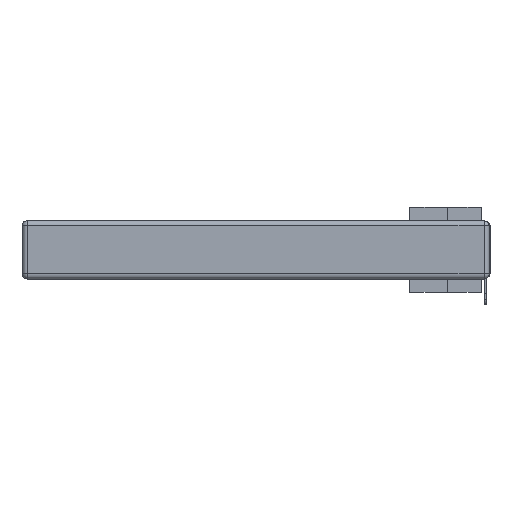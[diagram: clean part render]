
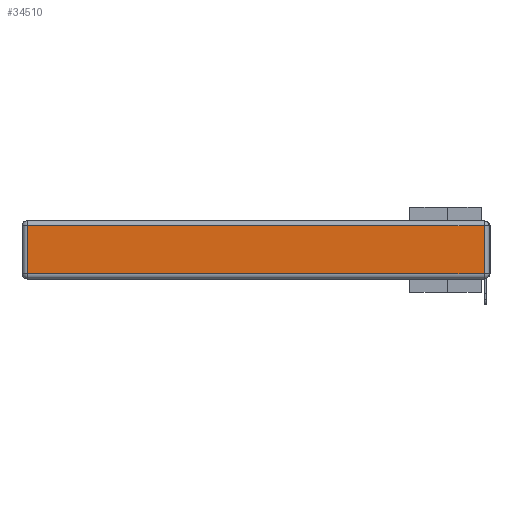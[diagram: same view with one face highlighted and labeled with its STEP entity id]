
A CAD part, left-side view. The second image highlights one B-rep face of the part: STEP entity #34510.
In plain terms, the highlighted planar face has unit normal (-1, 0, 0).
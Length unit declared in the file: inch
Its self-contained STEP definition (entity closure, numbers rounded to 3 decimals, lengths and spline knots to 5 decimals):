
#816 = DIRECTION ( 'NONE',  ( 0., 0., -1. ) ) ;
#1647 = VECTOR ( 'NONE', #14323, 39.37008 ) ;
#2009 = DIRECTION ( 'NONE',  ( 0., -1., 0. ) ) ;
#5439 = EDGE_LOOP ( 'NONE', ( #15310, #11260, #29568, #31312 ) ) ;
#5722 = EDGE_CURVE ( 'NONE', #29702, #23554, #7947, .T. ) ;
#7043 = EDGE_CURVE ( 'NONE', #12979, #22722, #29126, .T. ) ;
#7947 = LINE ( 'NONE', #18188, #13796 ) ;
#8484 = CARTESIAN_POINT ( 'NONE',  ( 0., 0.03, -0.03 ) ) ;
#8891 = CARTESIAN_POINT ( 'NONE',  ( 0., 0., -0.343 ) ) ;
#11260 = ORIENTED_EDGE ( 'NONE', *, *, #16206, .T. ) ;
#11688 = PLANE ( 'NONE',  #19322 ) ;
#12421 = LINE ( 'NONE', #22014, #30352 ) ;
#12979 = VERTEX_POINT ( 'NONE', #8484 ) ;
#13796 = VECTOR ( 'NONE', #2009, 39.37008 ) ;
#14323 = DIRECTION ( 'NONE',  ( 0., 0., 1. ) ) ;
#15310 = ORIENTED_EDGE ( 'NONE', *, *, #5722, .T. ) ;
#16206 = EDGE_CURVE ( 'NONE', #23554, #12979, #17492, .T. ) ;
#17492 = LINE ( 'NONE', #20139, #1647 ) ;
#18188 = CARTESIAN_POINT ( 'NONE',  ( 0., 0., -0.313 ) ) ;
#18224 = DIRECTION ( 'NONE',  ( 0., 1., 0. ) ) ;
#19322 = AXIS2_PLACEMENT_3D ( 'NONE', #8891, #24958, #27906 ) ;
#19706 = CARTESIAN_POINT ( 'NONE',  ( 0., 0.03, -0.313 ) ) ;
#20139 = CARTESIAN_POINT ( 'NONE',  ( 0., 0.03, -0.343 ) ) ;
#22014 = CARTESIAN_POINT ( 'NONE',  ( 0., 2.72, -0.343 ) ) ;
#22503 = FACE_OUTER_BOUND ( 'NONE', #5439, .T. ) ;
#22722 = VERTEX_POINT ( 'NONE', #32168 ) ;
#23554 = VERTEX_POINT ( 'NONE', #19706 ) ;
#23624 = EDGE_CURVE ( 'NONE', #22722, #29702, #12421, .T. ) ;
#23681 = VECTOR ( 'NONE', #18224, 39.37008 ) ;
#24958 = DIRECTION ( 'NONE',  ( -1., 0., 0. ) ) ;
#27906 = DIRECTION ( 'NONE',  ( 0., 0., 1. ) ) ;
#29083 = CARTESIAN_POINT ( 'NONE',  ( 0., 2.75, -0.03 ) ) ;
#29126 = LINE ( 'NONE', #29083, #23681 ) ;
#29471 = CARTESIAN_POINT ( 'NONE',  ( 0., 2.72, -0.313 ) ) ;
#29568 = ORIENTED_EDGE ( 'NONE', *, *, #7043, .T. ) ;
#29702 = VERTEX_POINT ( 'NONE', #29471 ) ;
#30352 = VECTOR ( 'NONE', #816, 39.37008 ) ;
#31312 = ORIENTED_EDGE ( 'NONE', *, *, #23624, .T. ) ;
#32168 = CARTESIAN_POINT ( 'NONE',  ( 0., 2.72, -0.03 ) ) ;
#34510 = ADVANCED_FACE ( 'NONE', ( #22503 ), #11688, .T. ) ;
